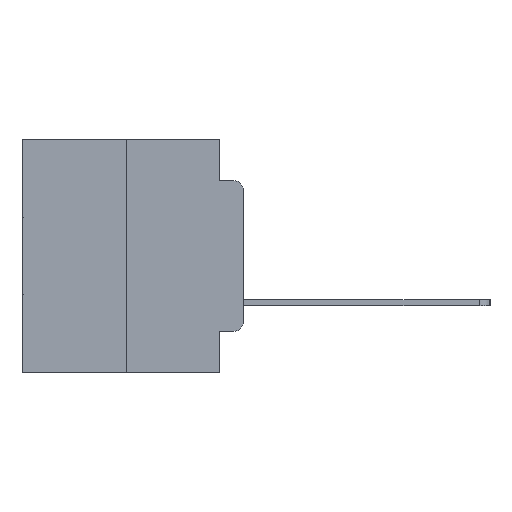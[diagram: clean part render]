
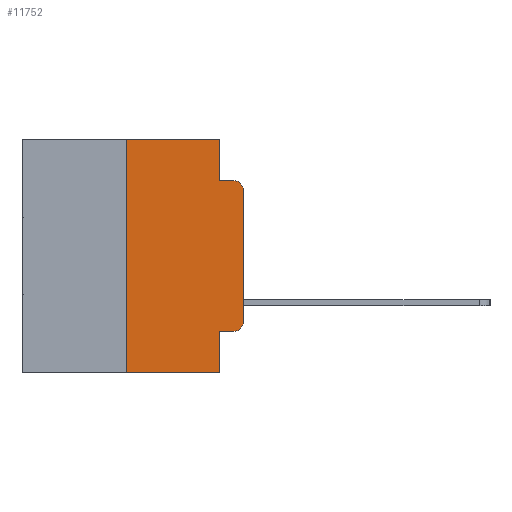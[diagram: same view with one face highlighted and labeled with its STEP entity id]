
A CAD part, left-side view. The second image highlights one B-rep face of the part: STEP entity #11752.
In plain terms, the highlighted planar face has unit normal (-1, 0, 0).
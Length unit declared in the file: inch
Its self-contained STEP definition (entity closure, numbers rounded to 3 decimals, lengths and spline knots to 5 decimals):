
#19 = VERTEX_POINT ( 'NONE', #18867 ) ;
#94 = VECTOR ( 'NONE', #1296, 39.37008 ) ;
#452 = VERTEX_POINT ( 'NONE', #3664 ) ;
#758 = EDGE_LOOP ( 'NONE', ( #10180, #10352, #11324, #12083, #24955, #14016, #14098, #16750, #19334, #18619 ) ) ;
#887 = DIRECTION ( 'NONE',  ( 0., 0., 1. ) ) ;
#1084 = VECTOR ( 'NONE', #15013, 39.37008 ) ;
#1274 = EDGE_CURVE ( 'NONE', #14276, #452, #29533, .T. ) ;
#1296 = DIRECTION ( 'NONE',  ( 0., -1., 0. ) ) ;
#1624 = VERTEX_POINT ( 'NONE', #3803 ) ;
#2431 = VERTEX_POINT ( 'NONE', #15873 ) ;
#3513 = LINE ( 'NONE', #20427, #15063 ) ;
#3565 = CARTESIAN_POINT ( 'NONE',  ( 0., 0.25, 0. ) ) ;
#3615 = LINE ( 'NONE', #29470, #28557 ) ;
#3664 = CARTESIAN_POINT ( 'NONE',  ( 0., 0.02, -0.0885 ) ) ;
#3803 = CARTESIAN_POINT ( 'NONE',  ( 0., 0.02, -0.4115 ) ) ;
#3965 = CIRCLE ( 'NONE', #27480, 0.02 ) ;
#4024 = CARTESIAN_POINT ( 'NONE',  ( 0., 0., 0. ) ) ;
#4357 = EDGE_CURVE ( 'NONE', #19, #14276, #14727, .T. ) ;
#6243 = CARTESIAN_POINT ( 'NONE',  ( 0., 0.25, -0.5 ) ) ;
#6526 = LINE ( 'NONE', #17397, #1084 ) ;
#7159 = CARTESIAN_POINT ( 'NONE',  ( 0., 0.02, -0.3915 ) ) ;
#8151 = CARTESIAN_POINT ( 'NONE',  ( 0., 0.051, -0.0885 ) ) ;
#9116 = DIRECTION ( 'NONE',  ( 0., 0., -1. ) ) ;
#9415 = EDGE_CURVE ( 'NONE', #9895, #9805, #3615, .T. ) ;
#9471 = DIRECTION ( 'NONE',  ( 0., 0., -1. ) ) ;
#9491 = LINE ( 'NONE', #28217, #15609 ) ;
#9805 = VERTEX_POINT ( 'NONE', #28589 ) ;
#9895 = VERTEX_POINT ( 'NONE', #6243 ) ;
#10180 = ORIENTED_EDGE ( 'NONE', *, *, #4357, .T. ) ;
#10352 = ORIENTED_EDGE ( 'NONE', *, *, #1274, .T. ) ;
#10402 = VERTEX_POINT ( 'NONE', #3565 ) ;
#10674 = FACE_OUTER_BOUND ( 'NONE', #758, .T. ) ;
#10783 = PLANE ( 'NONE',  #29342 ) ;
#11029 = CARTESIAN_POINT ( 'NONE',  ( 0., 0., -0.1085 ) ) ;
#11324 = ORIENTED_EDGE ( 'NONE', *, *, #27832, .F. ) ;
#11343 = CARTESIAN_POINT ( 'NONE',  ( 0., 0.051, -0.4115 ) ) ;
#11752 = ADVANCED_FACE ( 'NONE', ( #10674 ), #10783, .F. ) ;
#11768 = CARTESIAN_POINT ( 'NONE',  ( 0., 0.02, -0.1085 ) ) ;
#12083 = ORIENTED_EDGE ( 'NONE', *, *, #24862, .F. ) ;
#13019 = CARTESIAN_POINT ( 'NONE',  ( 0., 0.473, 0. ) ) ;
#13115 = DIRECTION ( 'NONE',  ( 0., 0., -1. ) ) ;
#13715 = VECTOR ( 'NONE', #9116, 39.37008 ) ;
#13724 = DIRECTION ( 'NONE',  ( 0., -1., 0. ) ) ;
#14016 = ORIENTED_EDGE ( 'NONE', *, *, #23362, .F. ) ;
#14098 = ORIENTED_EDGE ( 'NONE', *, *, #9415, .T. ) ;
#14126 = DIRECTION ( 'NONE',  ( 0., 0., -1. ) ) ;
#14276 = VERTEX_POINT ( 'NONE', #11029 ) ;
#14440 = LINE ( 'NONE', #24957, #13715 ) ;
#14727 = LINE ( 'NONE', #4024, #20056 ) ;
#15013 = DIRECTION ( 'NONE',  ( 0., -1., 0. ) ) ;
#15063 = VECTOR ( 'NONE', #22701, 39.37008 ) ;
#15535 = DIRECTION ( 'NONE',  ( 0., 0., 1. ) ) ;
#15609 = VECTOR ( 'NONE', #887, 39.37008 ) ;
#15762 = EDGE_CURVE ( 'NONE', #1624, #19, #3965, .T. ) ;
#15873 = CARTESIAN_POINT ( 'NONE',  ( 0., 0.051, 0. ) ) ;
#16642 = DIRECTION ( 'NONE',  ( 0., 0., -1. ) ) ;
#16750 = ORIENTED_EDGE ( 'NONE', *, *, #20310, .F. ) ;
#17277 = EDGE_CURVE ( 'NONE', #26258, #1624, #6526, .T. ) ;
#17397 = CARTESIAN_POINT ( 'NONE',  ( 0., 0.051, -0.4115 ) ) ;
#17429 = VERTEX_POINT ( 'NONE', #8151 ) ;
#18400 = AXIS2_PLACEMENT_3D ( 'NONE', #11768, #27647, #14126 ) ;
#18619 = ORIENTED_EDGE ( 'NONE', *, *, #15762, .T. ) ;
#18867 = CARTESIAN_POINT ( 'NONE',  ( 0., 0., -0.3915 ) ) ;
#18895 = CARTESIAN_POINT ( 'NONE',  ( 0., 0.051, 0. ) ) ;
#19211 = LINE ( 'NONE', #28600, #94 ) ;
#19334 = ORIENTED_EDGE ( 'NONE', *, *, #17277, .T. ) ;
#19398 = EDGE_CURVE ( 'NONE', #10402, #2431, #3513, .T. ) ;
#20056 = VECTOR ( 'NONE', #15535, 39.37008 ) ;
#20310 = EDGE_CURVE ( 'NONE', #26258, #9805, #26339, .T. ) ;
#20427 = CARTESIAN_POINT ( 'NONE',  ( 0., 0.473, 0. ) ) ;
#22701 = DIRECTION ( 'NONE',  ( 0., -1., 0. ) ) ;
#23144 = DIRECTION ( 'NONE',  ( -1., 0., 0. ) ) ;
#23362 = EDGE_CURVE ( 'NONE', #9895, #10402, #9491, .T. ) ;
#24862 = EDGE_CURVE ( 'NONE', #2431, #17429, #14440, .T. ) ;
#24955 = ORIENTED_EDGE ( 'NONE', *, *, #19398, .F. ) ;
#24957 = CARTESIAN_POINT ( 'NONE',  ( 0., 0.051, 0. ) ) ;
#25635 = VECTOR ( 'NONE', #16642, 39.37008 ) ;
#26258 = VERTEX_POINT ( 'NONE', #11343 ) ;
#26339 = LINE ( 'NONE', #18895, #25635 ) ;
#26679 = DIRECTION ( 'NONE',  ( 1., 0., 0. ) ) ;
#27480 = AXIS2_PLACEMENT_3D ( 'NONE', #7159, #23144, #9471 ) ;
#27647 = DIRECTION ( 'NONE',  ( -1., 0., 0. ) ) ;
#27832 = EDGE_CURVE ( 'NONE', #17429, #452, #19211, .T. ) ;
#28217 = CARTESIAN_POINT ( 'NONE',  ( 0., 0.25, 0. ) ) ;
#28557 = VECTOR ( 'NONE', #13724, 39.37008 ) ;
#28589 = CARTESIAN_POINT ( 'NONE',  ( 0., 0.051, -0.5 ) ) ;
#28600 = CARTESIAN_POINT ( 'NONE',  ( 0., 0.051, -0.0885 ) ) ;
#29342 = AXIS2_PLACEMENT_3D ( 'NONE', #13019, #26679, #13115 ) ;
#29470 = CARTESIAN_POINT ( 'NONE',  ( 0., 0.473, -0.5 ) ) ;
#29533 = CIRCLE ( 'NONE', #18400, 0.02 ) ;
